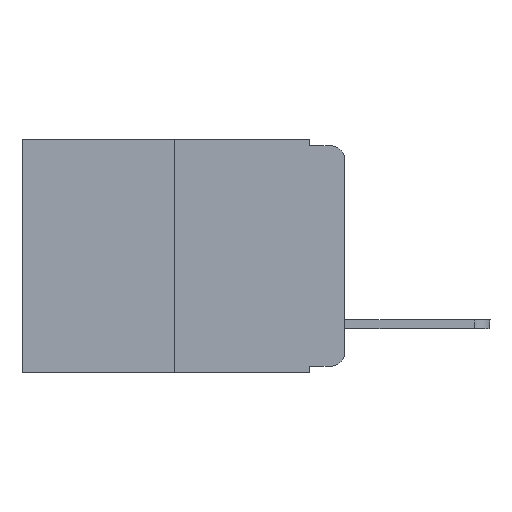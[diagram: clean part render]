
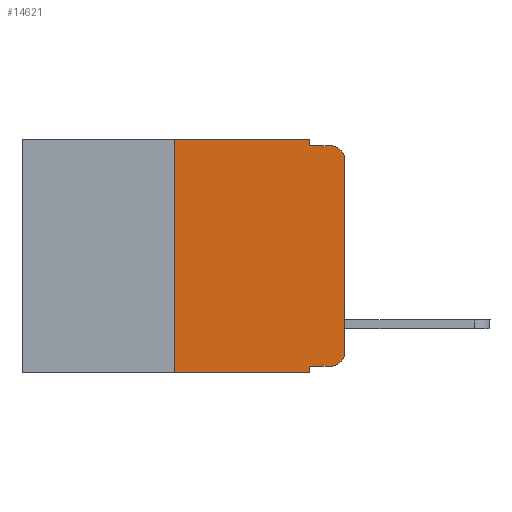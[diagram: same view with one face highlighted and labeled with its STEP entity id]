
A CAD part, left-side view. The second image highlights one B-rep face of the part: STEP entity #14621.
In plain terms, the highlighted planar face has unit normal (-1, 0, 0).
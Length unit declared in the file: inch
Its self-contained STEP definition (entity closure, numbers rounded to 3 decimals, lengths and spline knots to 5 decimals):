
#172 = VERTEX_POINT ( 'NONE', #2094 ) ;
#201 = CIRCLE ( 'NONE', #10967, 0.02 ) ;
#288 = CARTESIAN_POINT ( 'NONE',  ( 0., 0., -0.03 ) ) ;
#705 = CARTESIAN_POINT ( 'NONE',  ( 0., 0., 0. ) ) ;
#736 = ORIENTED_EDGE ( 'NONE', *, *, #3809, .F. ) ;
#938 = ORIENTED_EDGE ( 'NONE', *, *, #2875, .F. ) ;
#1027 = DIRECTION ( 'NONE',  ( 1., 0., 0. ) ) ;
#1659 = DIRECTION ( 'NONE',  ( 0., 0., -1. ) ) ;
#1921 = VERTEX_POINT ( 'NONE', #2815 ) ;
#1965 = ORIENTED_EDGE ( 'NONE', *, *, #3603, .T. ) ;
#2094 = CARTESIAN_POINT ( 'NONE',  ( 0., 0.051, -0.333 ) ) ;
#2157 = EDGE_CURVE ( 'NONE', #2938, #6703, #3704, .T. ) ;
#2208 = VECTOR ( 'NONE', #9554, 39.37008 ) ;
#2220 = CARTESIAN_POINT ( 'NONE',  ( 0., 0.473, -0.343 ) ) ;
#2428 = EDGE_CURVE ( 'NONE', #172, #9061, #4988, .T. ) ;
#2578 = CIRCLE ( 'NONE', #2624, 0.02 ) ;
#2624 = AXIS2_PLACEMENT_3D ( 'NONE', #5466, #4337, #6883 ) ;
#2815 = CARTESIAN_POINT ( 'NONE',  ( 0., 0.051, -0.01 ) ) ;
#2838 = ORIENTED_EDGE ( 'NONE', *, *, #3520, .T. ) ;
#2854 = CARTESIAN_POINT ( 'NONE',  ( 0., 0.25, 0. ) ) ;
#2875 = EDGE_CURVE ( 'NONE', #13504, #2938, #12700, .T. ) ;
#2938 = VERTEX_POINT ( 'NONE', #7047 ) ;
#3072 = ORIENTED_EDGE ( 'NONE', *, *, #11407, .T. ) ;
#3349 = CARTESIAN_POINT ( 'NONE',  ( 0., 0.25, -0.343 ) ) ;
#3477 = EDGE_CURVE ( 'NONE', #13504, #9061, #11550, .T. ) ;
#3520 = EDGE_CURVE ( 'NONE', #11755, #8467, #201, .T. ) ;
#3603 = EDGE_CURVE ( 'NONE', #13082, #7011, #2578, .T. ) ;
#3677 = CARTESIAN_POINT ( 'NONE',  ( 0., 0.051, 0. ) ) ;
#3704 = LINE ( 'NONE', #5480, #4072 ) ;
#3809 = EDGE_CURVE ( 'NONE', #6703, #1921, #13203, .T. ) ;
#4072 = VECTOR ( 'NONE', #6662, 39.37008 ) ;
#4080 = VECTOR ( 'NONE', #4411, 39.37008 ) ;
#4235 = ORIENTED_EDGE ( 'NONE', *, *, #9520, .F. ) ;
#4337 = DIRECTION ( 'NONE',  ( -1., 0., 0. ) ) ;
#4411 = DIRECTION ( 'NONE',  ( 0., 0., 1. ) ) ;
#4889 = LINE ( 'NONE', #5809, #14784 ) ;
#4973 = CARTESIAN_POINT ( 'NONE',  ( 0., 0.051, 0. ) ) ;
#4988 = LINE ( 'NONE', #3677, #11243 ) ;
#5466 = CARTESIAN_POINT ( 'NONE',  ( 0., 0.02, -0.313 ) ) ;
#5480 = CARTESIAN_POINT ( 'NONE',  ( 0., 0.473, 0. ) ) ;
#5758 = DIRECTION ( 'NONE',  ( 0., -1., 0. ) ) ;
#5778 = CARTESIAN_POINT ( 'NONE',  ( 0., 0.473, 0. ) ) ;
#5809 = CARTESIAN_POINT ( 'NONE',  ( 0., 0.051, -0.333 ) ) ;
#6618 = VECTOR ( 'NONE', #9719, 39.37008 ) ;
#6662 = DIRECTION ( 'NONE',  ( 0., -1., 0. ) ) ;
#6703 = VERTEX_POINT ( 'NONE', #6706 ) ;
#6706 = CARTESIAN_POINT ( 'NONE',  ( 0., 0.051, 0. ) ) ;
#6883 = DIRECTION ( 'NONE',  ( 0., 0., -1. ) ) ;
#7011 = VERTEX_POINT ( 'NONE', #10871 ) ;
#7047 = CARTESIAN_POINT ( 'NONE',  ( 0., 0.25, 0. ) ) ;
#8467 = VERTEX_POINT ( 'NONE', #13760 ) ;
#8482 = CARTESIAN_POINT ( 'NONE',  ( 0., 0.02, -0.333 ) ) ;
#8854 = ORIENTED_EDGE ( 'NONE', *, *, #2157, .F. ) ;
#9061 = VERTEX_POINT ( 'NONE', #14790 ) ;
#9116 = DIRECTION ( 'NONE',  ( 0., -1., 0. ) ) ;
#9402 = EDGE_LOOP ( 'NONE', ( #3072, #2838, #4235, #736, #8854, #938, #10259, #14645, #12642, #1965 ) ) ;
#9520 = EDGE_CURVE ( 'NONE', #1921, #8467, #13897, .T. ) ;
#9554 = DIRECTION ( 'NONE',  ( 0., -1., 0. ) ) ;
#9622 = EDGE_CURVE ( 'NONE', #172, #13082, #4889, .T. ) ;
#9719 = DIRECTION ( 'NONE',  ( 0., 0., 1. ) ) ;
#9807 = DIRECTION ( 'NONE',  ( -1., 0., 0. ) ) ;
#9909 = VECTOR ( 'NONE', #14246, 39.37008 ) ;
#10259 = ORIENTED_EDGE ( 'NONE', *, *, #3477, .T. ) ;
#10871 = CARTESIAN_POINT ( 'NONE',  ( 0., 0., -0.313 ) ) ;
#10967 = AXIS2_PLACEMENT_3D ( 'NONE', #13325, #9807, #12043 ) ;
#11243 = VECTOR ( 'NONE', #1659, 39.37008 ) ;
#11407 = EDGE_CURVE ( 'NONE', #7011, #11755, #13827, .T. ) ;
#11550 = LINE ( 'NONE', #2220, #2208 ) ;
#11755 = VERTEX_POINT ( 'NONE', #288 ) ;
#12043 = DIRECTION ( 'NONE',  ( 0., 0., -1. ) ) ;
#12640 = CARTESIAN_POINT ( 'NONE',  ( 0., 0.051, -0.01 ) ) ;
#12642 = ORIENTED_EDGE ( 'NONE', *, *, #9622, .T. ) ;
#12700 = LINE ( 'NONE', #2854, #6618 ) ;
#12981 = VECTOR ( 'NONE', #9116, 39.37008 ) ;
#13082 = VERTEX_POINT ( 'NONE', #8482 ) ;
#13203 = LINE ( 'NONE', #4973, #9909 ) ;
#13325 = CARTESIAN_POINT ( 'NONE',  ( 0., 0.02, -0.03 ) ) ;
#13504 = VERTEX_POINT ( 'NONE', #3349 ) ;
#13760 = CARTESIAN_POINT ( 'NONE',  ( 0., 0.02, -0.01 ) ) ;
#13827 = LINE ( 'NONE', #705, #4080 ) ;
#13882 = DIRECTION ( 'NONE',  ( 0., 0., -1. ) ) ;
#13897 = LINE ( 'NONE', #12640, #12981 ) ;
#14069 = FACE_OUTER_BOUND ( 'NONE', #9402, .T. ) ;
#14160 = AXIS2_PLACEMENT_3D ( 'NONE', #5778, #1027, #13882 ) ;
#14246 = DIRECTION ( 'NONE',  ( 0., 0., -1. ) ) ;
#14621 = ADVANCED_FACE ( 'NONE', ( #14069 ), #15133, .F. ) ;
#14645 = ORIENTED_EDGE ( 'NONE', *, *, #2428, .F. ) ;
#14784 = VECTOR ( 'NONE', #5758, 39.37008 ) ;
#14790 = CARTESIAN_POINT ( 'NONE',  ( 0., 0.051, -0.343 ) ) ;
#15133 = PLANE ( 'NONE',  #14160 ) ;
